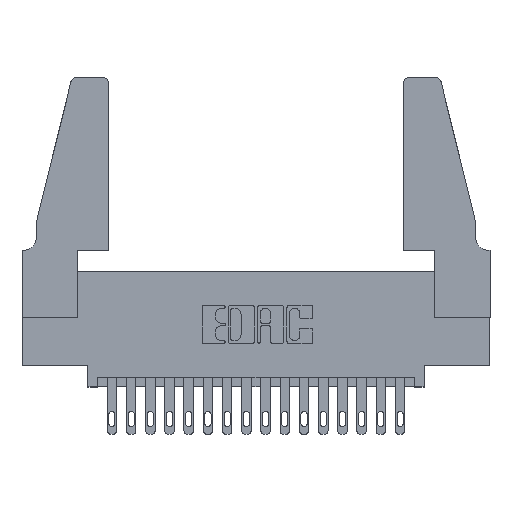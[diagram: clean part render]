
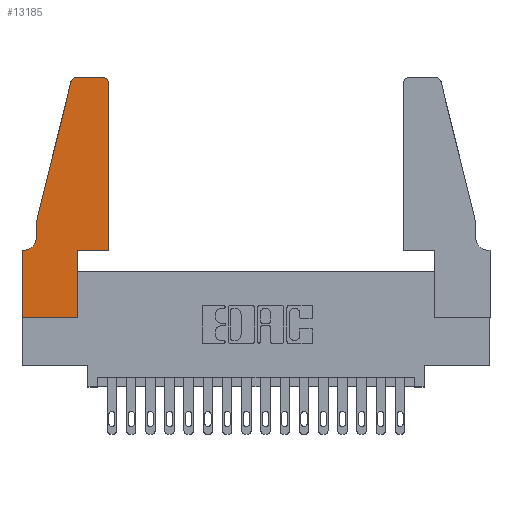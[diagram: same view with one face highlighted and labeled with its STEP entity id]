
A CAD part, top view. The second image highlights one B-rep face of the part: STEP entity #13185.
In plain terms, the highlighted planar face has unit normal (0, 0, 1).
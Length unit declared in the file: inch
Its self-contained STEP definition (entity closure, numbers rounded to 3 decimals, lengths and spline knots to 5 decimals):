
#181 = ORIENTED_EDGE ( 'NONE', *, *, #1100, .T. ) ;
#229 = CARTESIAN_POINT ( 'NONE',  ( 0.0755, 0.5, 0.37 ) ) ;
#714 = VECTOR ( 'NONE', #14420, 39.37008 ) ;
#717 = CARTESIAN_POINT ( 'NONE',  ( 0.0055, 0.35, 0.37 ) ) ;
#755 = EDGE_CURVE ( 'NONE', #2323, #12157, #12564, .T. ) ;
#785 = VERTEX_POINT ( 'NONE', #8114 ) ;
#905 = AXIS2_PLACEMENT_3D ( 'NONE', #14340, #12933, #17044 ) ;
#1033 = EDGE_CURVE ( 'NONE', #785, #6544, #7670, .T. ) ;
#1059 = CARTESIAN_POINT ( 'NONE',  ( 0.2865, 0., 0.37 ) ) ;
#1100 = EDGE_CURVE ( 'NONE', #6544, #2323, #8786, .T. ) ;
#1205 = EDGE_CURVE ( 'NONE', #11696, #12011, #13219, .T. ) ;
#1525 = VECTOR ( 'NONE', #2906, 39.37008 ) ;
#1708 = CIRCLE ( 'NONE', #10474, 0.03 ) ;
#1719 = VERTEX_POINT ( 'NONE', #7300 ) ;
#1735 = ORIENTED_EDGE ( 'NONE', *, *, #755, .T. ) ;
#1931 = CARTESIAN_POINT ( 'NONE',  ( 0.25487, 1.22718, 0.37 ) ) ;
#2146 = CARTESIAN_POINT ( 'NONE',  ( 0.0755, 0.5, 0.37 ) ) ;
#2317 = EDGE_CURVE ( 'NONE', #12206, #11595, #10891, .T. ) ;
#2323 = VERTEX_POINT ( 'NONE', #4868 ) ;
#2485 = LINE ( 'NONE', #2146, #3144 ) ;
#2510 = EDGE_CURVE ( 'NONE', #1719, #11696, #15770, .T. ) ;
#2672 = EDGE_CURVE ( 'NONE', #5073, #17715, #2485, .T. ) ;
#2906 = DIRECTION ( 'NONE',  ( 0., -1., 0. ) ) ;
#3144 = VECTOR ( 'NONE', #7782, 39.37008 ) ;
#3524 = VERTEX_POINT ( 'NONE', #15763 ) ;
#3837 = ORIENTED_EDGE ( 'NONE', *, *, #2510, .T. ) ;
#3903 = VECTOR ( 'NONE', #5544, 39.37008 ) ;
#4051 = CARTESIAN_POINT ( 'NONE',  ( 0.2605, 1.25, 0.37 ) ) ;
#4224 = DIRECTION ( 'NONE',  ( 1., 0., 0. ) ) ;
#4287 = ORIENTED_EDGE ( 'NONE', *, *, #1033, .T. ) ;
#4297 = PLANE ( 'NONE',  #13592 ) ;
#4868 = CARTESIAN_POINT ( 'NONE',  ( 0., 0.35, 0.37 ) ) ;
#5073 = VERTEX_POINT ( 'NONE', #1931 ) ;
#5133 = ORIENTED_EDGE ( 'NONE', *, *, #11649, .T. ) ;
#5544 = DIRECTION ( 'NONE',  ( -1., 0., 0. ) ) ;
#5561 = ORIENTED_EDGE ( 'NONE', *, *, #8591, .T. ) ;
#5750 = CARTESIAN_POINT ( 'NONE',  ( 0.2865, 0.35, 0.37 ) ) ;
#6134 = ORIENTED_EDGE ( 'NONE', *, *, #1205, .T. ) ;
#6544 = VERTEX_POINT ( 'NONE', #717 ) ;
#6678 = CARTESIAN_POINT ( 'NONE',  ( 0., 0., 0.37 ) ) ;
#6836 = DIRECTION ( 'NONE',  ( -1., 0., 0. ) ) ;
#6881 = DIRECTION ( 'NONE',  ( -1., 0., 0. ) ) ;
#7039 = DIRECTION ( 'NONE',  ( 0., 0., 1. ) ) ;
#7300 = CARTESIAN_POINT ( 'NONE',  ( 0.4505, 0.35, 0.37 ) ) ;
#7499 = ORIENTED_EDGE ( 'NONE', *, *, #2317, .T. ) ;
#7670 = CIRCLE ( 'NONE', #14550, 0.07 ) ;
#7697 = LINE ( 'NONE', #9573, #11023 ) ;
#7782 = DIRECTION ( 'NONE',  ( -0.239, -0.971, 0. ) ) ;
#8026 = DIRECTION ( 'NONE',  ( 1., 0., 0. ) ) ;
#8114 = CARTESIAN_POINT ( 'NONE',  ( 0.0755, 0.42, 0.37 ) ) ;
#8151 = VECTOR ( 'NONE', #4224, 39.37008 ) ;
#8174 = DIRECTION ( 'NONE',  ( 0., -1., 0. ) ) ;
#8479 = CARTESIAN_POINT ( 'NONE',  ( 0.0755, 0.35, 0.37 ) ) ;
#8591 = EDGE_CURVE ( 'NONE', #12011, #3524, #13347, .T. ) ;
#8786 = LINE ( 'NONE', #8479, #3903 ) ;
#9573 = CARTESIAN_POINT ( 'NONE',  ( 0.4505, 0.35, 0.37 ) ) ;
#9576 = VECTOR ( 'NONE', #6881, 39.37008 ) ;
#10308 = CARTESIAN_POINT ( 'NONE',  ( 0., 0.35, 0.37 ) ) ;
#10474 = AXIS2_PLACEMENT_3D ( 'NONE', #14308, #7039, #11276 ) ;
#10891 = LINE ( 'NONE', #5750, #17950 ) ;
#11023 = VECTOR ( 'NONE', #8026, 39.37008 ) ;
#11276 = DIRECTION ( 'NONE',  ( 1., 0., 0. ) ) ;
#11421 = CARTESIAN_POINT ( 'NONE',  ( 0.0755, 0.5, 0.37 ) ) ;
#11523 = DIRECTION ( 'NONE',  ( 0., 1., 0. ) ) ;
#11581 = EDGE_CURVE ( 'NONE', #11595, #1719, #7697, .T. ) ;
#11595 = VERTEX_POINT ( 'NONE', #18005 ) ;
#11626 = DIRECTION ( 'NONE',  ( 1., 0., 0. ) ) ;
#11649 = EDGE_CURVE ( 'NONE', #12157, #12206, #12807, .T. ) ;
#11696 = VERTEX_POINT ( 'NONE', #18198 ) ;
#11726 = LINE ( 'NONE', #229, #1525 ) ;
#11810 = DIRECTION ( 'NONE',  ( 0., 0., 1. ) ) ;
#12011 = VERTEX_POINT ( 'NONE', #16037 ) ;
#12157 = VERTEX_POINT ( 'NONE', #17986 ) ;
#12206 = VERTEX_POINT ( 'NONE', #1059 ) ;
#12287 = EDGE_CURVE ( 'NONE', #3524, #5073, #1708, .T. ) ;
#12324 = EDGE_LOOP ( 'NONE', ( #5561, #12894, #15710, #13203, #4287, #181, #1735, #5133, #7499, #13442, #3837, #6134 ) ) ;
#12332 = VECTOR ( 'NONE', #8174, 39.37008 ) ;
#12564 = LINE ( 'NONE', #6678, #12332 ) ;
#12807 = LINE ( 'NONE', #18249, #8151 ) ;
#12894 = ORIENTED_EDGE ( 'NONE', *, *, #12287, .T. ) ;
#12933 = DIRECTION ( 'NONE',  ( 0., 0., 1. ) ) ;
#13185 = ADVANCED_FACE ( 'NONE', ( #15829 ), #4297, .T. ) ;
#13203 = ORIENTED_EDGE ( 'NONE', *, *, #16745, .T. ) ;
#13219 = CIRCLE ( 'NONE', #905, 0.03 ) ;
#13347 = LINE ( 'NONE', #4051, #9576 ) ;
#13442 = ORIENTED_EDGE ( 'NONE', *, *, #11581, .T. ) ;
#13592 = AXIS2_PLACEMENT_3D ( 'NONE', #10308, #11810, #11626 ) ;
#13738 = DIRECTION ( 'NONE',  ( 0., 0., -1. ) ) ;
#14240 = CARTESIAN_POINT ( 'NONE',  ( 0.4505, 0.35, 0.37 ) ) ;
#14308 = CARTESIAN_POINT ( 'NONE',  ( 0.284, 1.22, 0.37 ) ) ;
#14340 = CARTESIAN_POINT ( 'NONE',  ( 0.4205, 1.22, 0.37 ) ) ;
#14420 = DIRECTION ( 'NONE',  ( 0., 1., 0. ) ) ;
#14550 = AXIS2_PLACEMENT_3D ( 'NONE', #17904, #13738, #6836 ) ;
#15710 = ORIENTED_EDGE ( 'NONE', *, *, #2672, .T. ) ;
#15763 = CARTESIAN_POINT ( 'NONE',  ( 0.284, 1.25, 0.37 ) ) ;
#15770 = LINE ( 'NONE', #14240, #714 ) ;
#15829 = FACE_OUTER_BOUND ( 'NONE', #12324, .T. ) ;
#16037 = CARTESIAN_POINT ( 'NONE',  ( 0.4205, 1.25, 0.37 ) ) ;
#16745 = EDGE_CURVE ( 'NONE', #17715, #785, #11726, .T. ) ;
#17044 = DIRECTION ( 'NONE',  ( 1., 0., 0. ) ) ;
#17715 = VERTEX_POINT ( 'NONE', #11421 ) ;
#17904 = CARTESIAN_POINT ( 'NONE',  ( 0.0055, 0.42, 0.37 ) ) ;
#17950 = VECTOR ( 'NONE', #11523, 39.37008 ) ;
#17986 = CARTESIAN_POINT ( 'NONE',  ( 0., 0., 0.37 ) ) ;
#18005 = CARTESIAN_POINT ( 'NONE',  ( 0.2865, 0.35, 0.37 ) ) ;
#18198 = CARTESIAN_POINT ( 'NONE',  ( 0.4505, 1.22, 0.37 ) ) ;
#18249 = CARTESIAN_POINT ( 'NONE',  ( 0., 0., 0.37 ) ) ;
